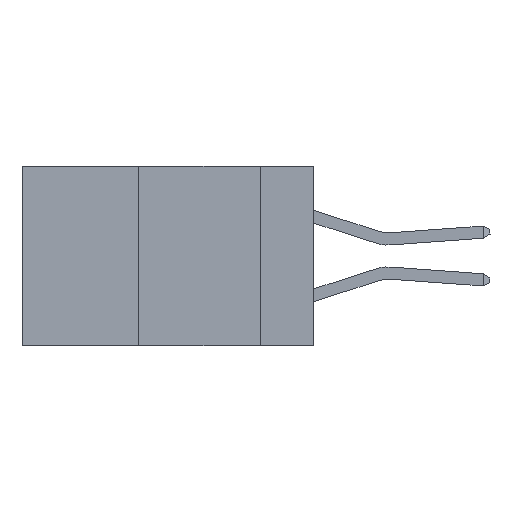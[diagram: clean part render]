
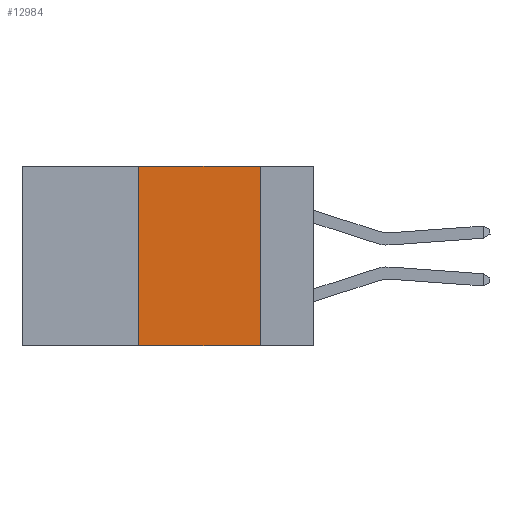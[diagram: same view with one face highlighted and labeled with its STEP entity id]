
A CAD part, left-side view. The second image highlights one B-rep face of the part: STEP entity #12984.
In plain terms, the highlighted planar face has unit normal (-1, 0, 0).
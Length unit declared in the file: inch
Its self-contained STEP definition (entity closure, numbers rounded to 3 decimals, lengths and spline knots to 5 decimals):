
#1452 = VERTEX_POINT ( 'NONE', #17806 ) ;
#1949 = CARTESIAN_POINT ( 'NONE',  ( 0., 0.6, 0. ) ) ;
#2538 = DIRECTION ( 'NONE',  ( 0., 0., -1. ) ) ;
#2567 = CARTESIAN_POINT ( 'NONE',  ( 0., 0.6, 0. ) ) ;
#2593 = ORIENTED_EDGE ( 'NONE', *, *, #10558, .F. ) ;
#2796 = LINE ( 'NONE', #24750, #18443 ) ;
#3749 = ORIENTED_EDGE ( 'NONE', *, *, #4764, .F. ) ;
#3794 = DIRECTION ( 'NONE',  ( 0., -1., 0. ) ) ;
#3922 = ORIENTED_EDGE ( 'NONE', *, *, #17351, .F. ) ;
#4066 = DIRECTION ( 'NONE',  ( 0., 0., -1. ) ) ;
#4196 = VECTOR ( 'NONE', #22448, 39.37008 ) ;
#4764 = EDGE_CURVE ( 'NONE', #13960, #15107, #18210, .T. ) ;
#6088 = VECTOR ( 'NONE', #8981, 39.37008 ) ;
#8981 = DIRECTION ( 'NONE',  ( 0., -1., 0. ) ) ;
#10326 = EDGE_CURVE ( 'NONE', #13960, #23586, #2796, .T. ) ;
#10402 = LINE ( 'NONE', #2567, #6088 ) ;
#10558 = EDGE_CURVE ( 'NONE', #15107, #1452, #10402, .T. ) ;
#12061 = CARTESIAN_POINT ( 'NONE',  ( 0., 0.36, -0.37 ) ) ;
#12578 = LINE ( 'NONE', #13300, #17957 ) ;
#12984 = ADVANCED_FACE ( 'NONE', ( #24185 ), #20996, .F. ) ;
#13063 = AXIS2_PLACEMENT_3D ( 'NONE', #1949, #16801, #4066 ) ;
#13300 = CARTESIAN_POINT ( 'NONE',  ( 0., 0.11, 0. ) ) ;
#13960 = VERTEX_POINT ( 'NONE', #12061 ) ;
#15107 = VERTEX_POINT ( 'NONE', #22046 ) ;
#16801 = DIRECTION ( 'NONE',  ( 1., 0., 0. ) ) ;
#17351 = EDGE_CURVE ( 'NONE', #1452, #23586, #12578, .T. ) ;
#17806 = CARTESIAN_POINT ( 'NONE',  ( 0., 0.11, 0. ) ) ;
#17957 = VECTOR ( 'NONE', #2538, 39.37008 ) ;
#18210 = LINE ( 'NONE', #18632, #4196 ) ;
#18279 = EDGE_LOOP ( 'NONE', ( #3922, #2593, #3749, #24772 ) ) ;
#18443 = VECTOR ( 'NONE', #3794, 39.37008 ) ;
#18632 = CARTESIAN_POINT ( 'NONE',  ( 0., 0.36, 0. ) ) ;
#20996 = PLANE ( 'NONE',  #13063 ) ;
#22046 = CARTESIAN_POINT ( 'NONE',  ( 0., 0.36, 0. ) ) ;
#22448 = DIRECTION ( 'NONE',  ( 0., 0., 1. ) ) ;
#23232 = CARTESIAN_POINT ( 'NONE',  ( 0., 0.11, -0.37 ) ) ;
#23586 = VERTEX_POINT ( 'NONE', #23232 ) ;
#24185 = FACE_OUTER_BOUND ( 'NONE', #18279, .T. ) ;
#24750 = CARTESIAN_POINT ( 'NONE',  ( 0., 0.6, -0.37 ) ) ;
#24772 = ORIENTED_EDGE ( 'NONE', *, *, #10326, .T. ) ;
